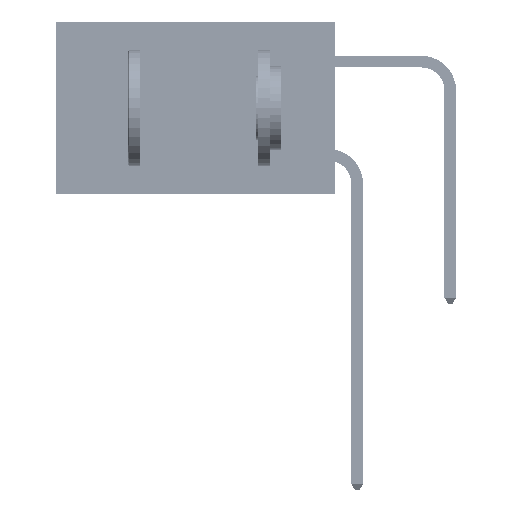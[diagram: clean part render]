
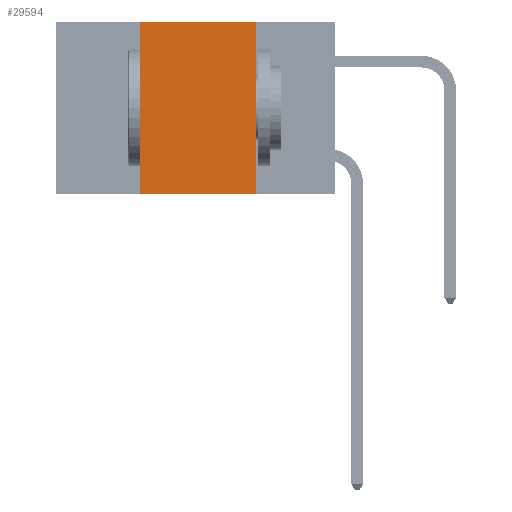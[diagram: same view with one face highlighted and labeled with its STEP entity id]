
A CAD part, left-side view. The second image highlights one B-rep face of the part: STEP entity #29594.
In plain terms, the highlighted planar face has unit normal (-1, 0, 0).
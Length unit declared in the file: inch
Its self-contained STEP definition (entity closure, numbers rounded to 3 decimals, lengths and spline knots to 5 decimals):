
#208 = LINE ( 'NONE', #21299, #31678 ) ;
#516 = VECTOR ( 'NONE', #18001, 39.37008 ) ;
#1504 = ORIENTED_EDGE ( 'NONE', *, *, #24949, .T. ) ;
#4524 = LINE ( 'NONE', #41239, #46809 ) ;
#5183 = EDGE_CURVE ( 'NONE', #33369, #44846, #5556, .T. ) ;
#5556 = LINE ( 'NONE', #28564, #27384 ) ;
#5858 = VERTEX_POINT ( 'NONE', #34805 ) ;
#11367 = FACE_OUTER_BOUND ( 'NONE', #15666, .T. ) ;
#11879 = DIRECTION ( 'NONE',  ( 0., -1., 0. ) ) ;
#13928 = CARTESIAN_POINT ( 'NONE',  ( 0., 0.6, -0.37 ) ) ;
#14602 = CARTESIAN_POINT ( 'NONE',  ( 0., 0.17, -0.37 ) ) ;
#14933 = DIRECTION ( 'NONE',  ( 0., 0., -1. ) ) ;
#15666 = EDGE_LOOP ( 'NONE', ( #47679, #39994, #41908, #1504 ) ) ;
#17283 = CARTESIAN_POINT ( 'NONE',  ( 0., 0.17, 0. ) ) ;
#18001 = DIRECTION ( 'NONE',  ( 0., -1., 0. ) ) ;
#18493 = LINE ( 'NONE', #13928, #516 ) ;
#21299 = CARTESIAN_POINT ( 'NONE',  ( 0., 0.42, 0. ) ) ;
#23937 = EDGE_CURVE ( 'NONE', #44846, #45078, #4524, .T. ) ;
#24949 = EDGE_CURVE ( 'NONE', #5858, #45078, #18493, .T. ) ;
#27141 = PLANE ( 'NONE',  #39409 ) ;
#27384 = VECTOR ( 'NONE', #11879, 39.37008 ) ;
#28564 = CARTESIAN_POINT ( 'NONE',  ( 0., 0.6, 0. ) ) ;
#29594 = ADVANCED_FACE ( 'NONE', ( #11367 ), #27141, .F. ) ;
#31678 = VECTOR ( 'NONE', #33496, 39.37008 ) ;
#33369 = VERTEX_POINT ( 'NONE', #51903 ) ;
#33496 = DIRECTION ( 'NONE',  ( 0., 0., 1. ) ) ;
#34805 = CARTESIAN_POINT ( 'NONE',  ( 0., 0.42, -0.37 ) ) ;
#39409 = AXIS2_PLACEMENT_3D ( 'NONE', #51530, #39441, #14933 ) ;
#39441 = DIRECTION ( 'NONE',  ( 1., 0., 0. ) ) ;
#39994 = ORIENTED_EDGE ( 'NONE', *, *, #5183, .F. ) ;
#41239 = CARTESIAN_POINT ( 'NONE',  ( 0., 0.17, 0. ) ) ;
#41908 = ORIENTED_EDGE ( 'NONE', *, *, #46892, .F. ) ;
#44846 = VERTEX_POINT ( 'NONE', #17283 ) ;
#45078 = VERTEX_POINT ( 'NONE', #14602 ) ;
#46809 = VECTOR ( 'NONE', #49415, 39.37008 ) ;
#46892 = EDGE_CURVE ( 'NONE', #5858, #33369, #208, .T. ) ;
#47679 = ORIENTED_EDGE ( 'NONE', *, *, #23937, .F. ) ;
#49415 = DIRECTION ( 'NONE',  ( 0., 0., -1. ) ) ;
#51530 = CARTESIAN_POINT ( 'NONE',  ( 0., 0.6, 0. ) ) ;
#51903 = CARTESIAN_POINT ( 'NONE',  ( 0., 0.42, 0. ) ) ;
